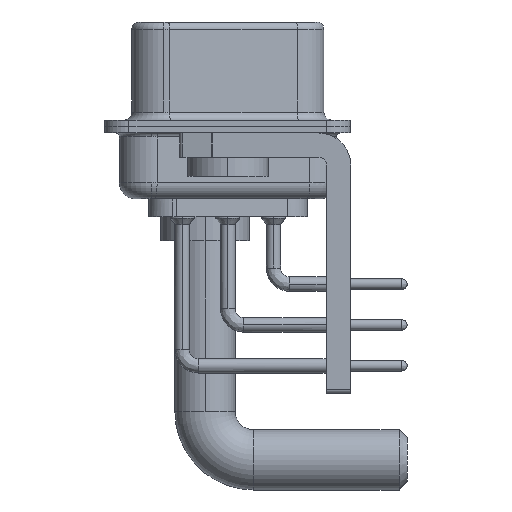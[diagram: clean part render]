
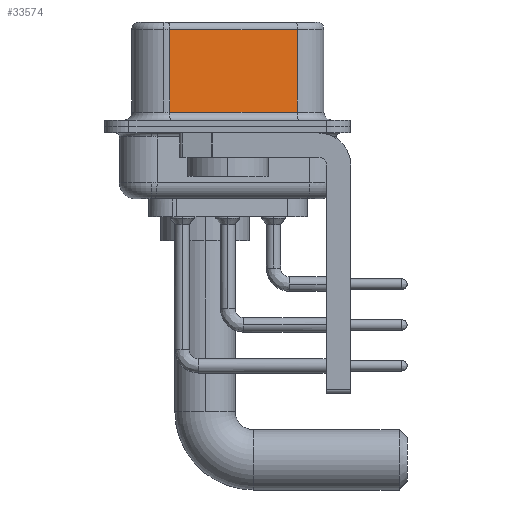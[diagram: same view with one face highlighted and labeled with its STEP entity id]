
A CAD part, left-side view. The second image highlights one B-rep face of the part: STEP entity #33574.
In plain terms, the highlighted planar face has unit normal (-0.985, -0.174, 0).
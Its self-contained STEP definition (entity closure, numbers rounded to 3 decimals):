
#1171 = LINE ( 'NONE', #36872, #9635 ) ;
#2181 = CARTESIAN_POINT ( 'NONE',  ( 3.73, 3.628, 0.9 ) ) ;
#2680 = CARTESIAN_POINT ( 'NONE',  ( 5.132, -4.322, 6.02 ) ) ;
#2879 = DIRECTION ( 'NONE',  ( -0.174, 0.985, 0. ) ) ;
#3551 = LINE ( 'NONE', #9354, #7175 ) ;
#4289 = DIRECTION ( 'NONE',  ( 0., 0., -1. ) ) ;
#4432 = ORIENTED_EDGE ( 'NONE', *, *, #7264, .T. ) ;
#6243 = VECTOR ( 'NONE', #2879, 1000. ) ;
#7175 = VECTOR ( 'NONE', #33366, 1000. ) ;
#7264 = EDGE_CURVE ( 'NONE', #20392, #20882, #17799, .T. ) ;
#7570 = DIRECTION ( 'NONE',  ( 0.174, -0.985, 0. ) ) ;
#9354 = CARTESIAN_POINT ( 'NONE',  ( 5.132, -4.322, 6.52 ) ) ;
#9510 = EDGE_CURVE ( 'NONE', #20392, #27685, #3551, .T. ) ;
#9635 = VECTOR ( 'NONE', #4289, 1000. ) ;
#9899 = ORIENTED_EDGE ( 'NONE', *, *, #19687, .T. ) ;
#12902 = DIRECTION ( 'NONE',  ( -0.174, 0.985, 0. ) ) ;
#13305 = VERTEX_POINT ( 'NONE', #2181 ) ;
#13713 = EDGE_CURVE ( 'NONE', #13305, #27685, #31585, .T. ) ;
#17799 = LINE ( 'NONE', #2680, #6243 ) ;
#18346 = PLANE ( 'NONE',  #37212 ) ;
#19687 = EDGE_CURVE ( 'NONE', #20882, #13305, #1171, .T. ) ;
#20063 = ORIENTED_EDGE ( 'NONE', *, *, #13713, .T. ) ;
#20392 = VERTEX_POINT ( 'NONE', #20522 ) ;
#20522 = CARTESIAN_POINT ( 'NONE',  ( 5.132, -4.322, 6.02 ) ) ;
#20882 = VERTEX_POINT ( 'NONE', #33601 ) ;
#22141 = CARTESIAN_POINT ( 'NONE',  ( 5.132, -4.322, 0.9 ) ) ;
#24912 = VECTOR ( 'NONE', #7570, 1000. ) ;
#27155 = ORIENTED_EDGE ( 'NONE', *, *, #9510, .F. ) ;
#27685 = VERTEX_POINT ( 'NONE', #22141 ) ;
#28024 = CARTESIAN_POINT ( 'NONE',  ( 5.132, -4.322, 6.52 ) ) ;
#28313 = CARTESIAN_POINT ( 'NONE',  ( 5.132, -4.322, 0.9 ) ) ;
#30168 = DIRECTION ( 'NONE',  ( 0.985, 0.174, 0. ) ) ;
#30352 = FACE_OUTER_BOUND ( 'NONE', #35511, .T. ) ;
#31585 = LINE ( 'NONE', #28313, #24912 ) ;
#33366 = DIRECTION ( 'NONE',  ( 0., 0., -1. ) ) ;
#33574 = ADVANCED_FACE ( 'NONE', ( #30352 ), #18346, .F. ) ;
#33601 = CARTESIAN_POINT ( 'NONE',  ( 3.73, 3.628, 6.02 ) ) ;
#35511 = EDGE_LOOP ( 'NONE', ( #27155, #4432, #9899, #20063 ) ) ;
#36872 = CARTESIAN_POINT ( 'NONE',  ( 3.73, 3.628, 6.52 ) ) ;
#37212 = AXIS2_PLACEMENT_3D ( 'NONE', #28024, #30168, #12902 ) ;
